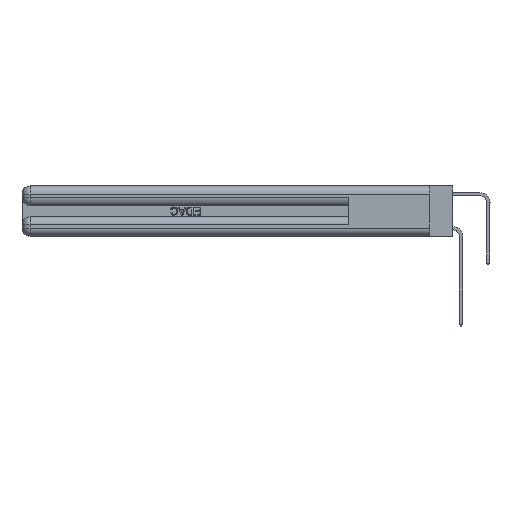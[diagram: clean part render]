
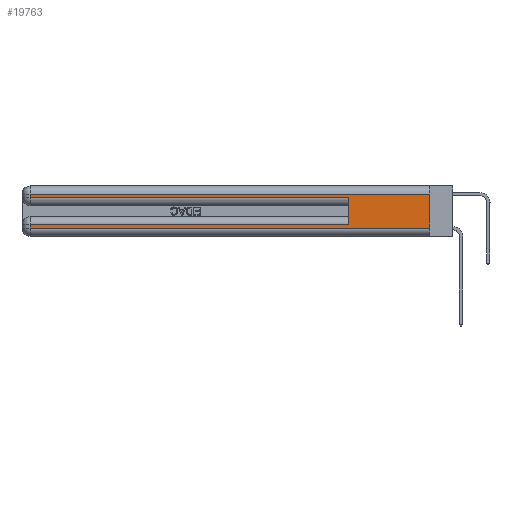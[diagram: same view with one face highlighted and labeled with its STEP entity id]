
A CAD part, left-side view. The second image highlights one B-rep face of the part: STEP entity #19763.
In plain terms, the highlighted planar face has unit normal (-1, 0, 0).
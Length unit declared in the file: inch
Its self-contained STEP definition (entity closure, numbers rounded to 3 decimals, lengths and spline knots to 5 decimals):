
#97 = VERTEX_POINT ( 'NONE', #30601 ) ;
#494 = EDGE_CURVE ( 'NONE', #97, #13401, #17869, .T. ) ;
#575 = DIRECTION ( 'NONE',  ( 0., -1., 0. ) ) ;
#1095 = EDGE_CURVE ( 'NONE', #18582, #35059, #31553, .T. ) ;
#2186 = DIRECTION ( 'NONE',  ( 0., 0., -1. ) ) ;
#2886 = VECTOR ( 'NONE', #8909, 39.37008 ) ;
#3147 = CARTESIAN_POINT ( 'NONE',  ( 0., 0., 0.31 ) ) ;
#3661 = ORIENTED_EDGE ( 'NONE', *, *, #35208, .T. ) ;
#3671 = VERTEX_POINT ( 'NONE', #10314 ) ;
#3920 = VERTEX_POINT ( 'NONE', #19033 ) ;
#4164 = LINE ( 'NONE', #15027, #25795 ) ;
#4220 = VERTEX_POINT ( 'NONE', #17752 ) ;
#4512 = CARTESIAN_POINT ( 'NONE',  ( 0., 0.6, 0.285 ) ) ;
#4916 = DIRECTION ( 'NONE',  ( 1., 0., 0. ) ) ;
#4987 = CARTESIAN_POINT ( 'NONE',  ( 0., 2.94, 0.06 ) ) ;
#5220 = ORIENTED_EDGE ( 'NONE', *, *, #494, .F. ) ;
#5905 = AXIS2_PLACEMENT_3D ( 'NONE', #21455, #4916, #2186 ) ;
#5932 = EDGE_LOOP ( 'NONE', ( #7751, #28988, #17831, #10119, #5220, #3661, #35935, #29184 ) ) ;
#7751 = ORIENTED_EDGE ( 'NONE', *, *, #14984, .F. ) ;
#8909 = DIRECTION ( 'NONE',  ( 0., 0., 1. ) ) ;
#9111 = CARTESIAN_POINT ( 'NONE',  ( 0., 2.94, 0.37 ) ) ;
#10119 = ORIENTED_EDGE ( 'NONE', *, *, #30037, .T. ) ;
#10145 = DIRECTION ( 'NONE',  ( 0., 0., -1. ) ) ;
#10314 = CARTESIAN_POINT ( 'NONE',  ( 0., 2.94, 0.285 ) ) ;
#13401 = VERTEX_POINT ( 'NONE', #4512 ) ;
#14938 = VECTOR ( 'NONE', #575, 39.37008 ) ;
#14984 = EDGE_CURVE ( 'NONE', #18582, #3920, #30669, .T. ) ;
#15027 = CARTESIAN_POINT ( 'NONE',  ( 0., 0., 0.285 ) ) ;
#15323 = EDGE_CURVE ( 'NONE', #20170, #3920, #16694, .T. ) ;
#15334 = LINE ( 'NONE', #33867, #20623 ) ;
#16297 = CARTESIAN_POINT ( 'NONE',  ( 0., 2.94, 0.31 ) ) ;
#16694 = LINE ( 'NONE', #17697, #14938 ) ;
#17101 = LINE ( 'NONE', #35884, #29062 ) ;
#17697 = CARTESIAN_POINT ( 'NONE',  ( 0., 0., 0.06 ) ) ;
#17752 = CARTESIAN_POINT ( 'NONE',  ( 0., 2.94, 0.085 ) ) ;
#17831 = ORIENTED_EDGE ( 'NONE', *, *, #24090, .T. ) ;
#17869 = LINE ( 'NONE', #28712, #2886 ) ;
#18582 = VERTEX_POINT ( 'NONE', #3147 ) ;
#19033 = CARTESIAN_POINT ( 'NONE',  ( 0., 0., 0.06 ) ) ;
#19059 = PLANE ( 'NONE',  #5905 ) ;
#19122 = VECTOR ( 'NONE', #34536, 39.37008 ) ;
#19763 = ADVANCED_FACE ( 'NONE', ( #29229 ), #19059, .F. ) ;
#20170 = VERTEX_POINT ( 'NONE', #4987 ) ;
#20482 = VECTOR ( 'NONE', #21658, 39.37008 ) ;
#20558 = LINE ( 'NONE', #9111, #32515 ) ;
#20623 = VECTOR ( 'NONE', #31461, 39.37008 ) ;
#20723 = DIRECTION ( 'NONE',  ( 0., 0., -1. ) ) ;
#21455 = CARTESIAN_POINT ( 'NONE',  ( 0., 0., 0.37 ) ) ;
#21658 = DIRECTION ( 'NONE',  ( 0., 1., 0. ) ) ;
#23115 = CARTESIAN_POINT ( 'NONE',  ( 0., 0., 0.37 ) ) ;
#23292 = DIRECTION ( 'NONE',  ( 0., -1., 0. ) ) ;
#24090 = EDGE_CURVE ( 'NONE', #35059, #3671, #20558, .T. ) ;
#25795 = VECTOR ( 'NONE', #23292, 39.37008 ) ;
#28712 = CARTESIAN_POINT ( 'NONE',  ( 0., 0.6, 0.145 ) ) ;
#28988 = ORIENTED_EDGE ( 'NONE', *, *, #1095, .T. ) ;
#29062 = VECTOR ( 'NONE', #10145, 39.37008 ) ;
#29184 = ORIENTED_EDGE ( 'NONE', *, *, #15323, .T. ) ;
#29229 = FACE_OUTER_BOUND ( 'NONE', #5932, .T. ) ;
#30037 = EDGE_CURVE ( 'NONE', #3671, #13401, #4164, .T. ) ;
#30601 = CARTESIAN_POINT ( 'NONE',  ( 0., 0.6, 0.085 ) ) ;
#30669 = LINE ( 'NONE', #23115, #19122 ) ;
#31461 = DIRECTION ( 'NONE',  ( 0., 1., 0. ) ) ;
#31553 = LINE ( 'NONE', #32685, #20482 ) ;
#32515 = VECTOR ( 'NONE', #20723, 39.37008 ) ;
#32685 = CARTESIAN_POINT ( 'NONE',  ( 0., 0., 0.31 ) ) ;
#33867 = CARTESIAN_POINT ( 'NONE',  ( 0., 0., 0.085 ) ) ;
#34536 = DIRECTION ( 'NONE',  ( 0., 0., -1. ) ) ;
#34880 = EDGE_CURVE ( 'NONE', #4220, #20170, #17101, .T. ) ;
#35059 = VERTEX_POINT ( 'NONE', #16297 ) ;
#35208 = EDGE_CURVE ( 'NONE', #97, #4220, #15334, .T. ) ;
#35884 = CARTESIAN_POINT ( 'NONE',  ( 0., 2.94, 0.37 ) ) ;
#35935 = ORIENTED_EDGE ( 'NONE', *, *, #34880, .T. ) ;
